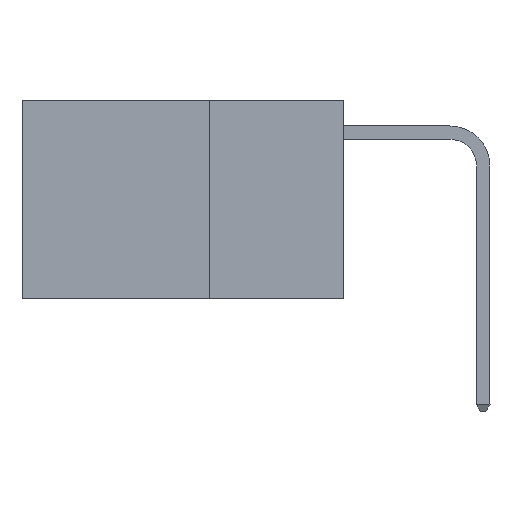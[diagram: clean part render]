
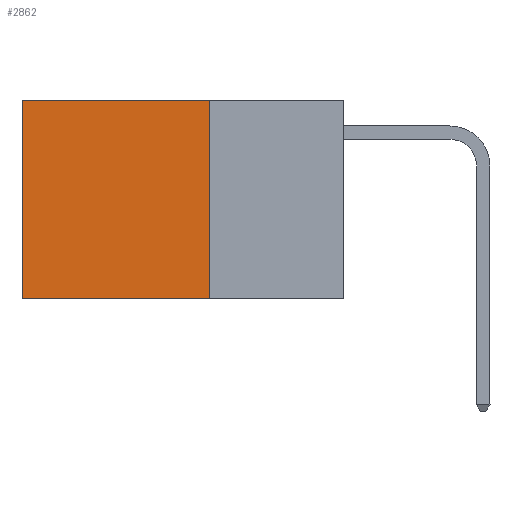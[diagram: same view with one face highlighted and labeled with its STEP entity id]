
A CAD part, left-side view. The second image highlights one B-rep face of the part: STEP entity #2862.
In plain terms, the highlighted planar face has unit normal (-1, 0, 0).
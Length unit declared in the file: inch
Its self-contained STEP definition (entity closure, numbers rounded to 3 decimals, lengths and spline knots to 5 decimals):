
#865 = CARTESIAN_POINT ( 'NONE',  ( 0.2625, 0.6, 0. ) ) ;
#990 = VECTOR ( 'NONE', #8716, 39.37008 ) ;
#1269 = VERTEX_POINT ( 'NONE', #865 ) ;
#1334 = VERTEX_POINT ( 'NONE', #7716 ) ;
#2862 = ADVANCED_FACE ( 'NONE', ( #6163 ), #12573, .F. ) ;
#3674 = EDGE_LOOP ( 'NONE', ( #12179, #13144, #6702, #9783 ) ) ;
#3765 = EDGE_CURVE ( 'NONE', #15240, #1334, #6272, .T. ) ;
#4003 = EDGE_CURVE ( 'NONE', #10254, #1269, #8808, .T. ) ;
#4923 = CARTESIAN_POINT ( 'NONE',  ( 0.2625, 0.25, -0.37 ) ) ;
#5014 = DIRECTION ( 'NONE',  ( 0., 1., 0. ) ) ;
#5397 = VECTOR ( 'NONE', #5014, 39.37008 ) ;
#5686 = LINE ( 'NONE', #14625, #9878 ) ;
#6163 = FACE_OUTER_BOUND ( 'NONE', #3674, .T. ) ;
#6244 = DIRECTION ( 'NONE',  ( 1., 0., 0. ) ) ;
#6272 = LINE ( 'NONE', #4923, #5397 ) ;
#6702 = ORIENTED_EDGE ( 'NONE', *, *, #14490, .F. ) ;
#7448 = CARTESIAN_POINT ( 'NONE',  ( 0.2625, 0.25, 0. ) ) ;
#7615 = DIRECTION ( 'NONE',  ( 0., 0., -1. ) ) ;
#7716 = CARTESIAN_POINT ( 'NONE',  ( 0.2625, 0.6, -0.37 ) ) ;
#8716 = DIRECTION ( 'NONE',  ( 0., 1., 0. ) ) ;
#8808 = LINE ( 'NONE', #13926, #990 ) ;
#9783 = ORIENTED_EDGE ( 'NONE', *, *, #4003, .T. ) ;
#9863 = DIRECTION ( 'NONE',  ( 0., 0., -1. ) ) ;
#9878 = VECTOR ( 'NONE', #13215, 39.37008 ) ;
#10254 = VERTEX_POINT ( 'NONE', #10658 ) ;
#10658 = CARTESIAN_POINT ( 'NONE',  ( 0.2625, 0.25, 0. ) ) ;
#10782 = VECTOR ( 'NONE', #9863, 39.37008 ) ;
#10873 = AXIS2_PLACEMENT_3D ( 'NONE', #7448, #6244, #7615 ) ;
#11032 = EDGE_CURVE ( 'NONE', #1269, #1334, #5686, .T. ) ;
#12179 = ORIENTED_EDGE ( 'NONE', *, *, #11032, .T. ) ;
#12220 = CARTESIAN_POINT ( 'NONE',  ( 0.2625, 0.25, 0. ) ) ;
#12573 = PLANE ( 'NONE',  #10873 ) ;
#13144 = ORIENTED_EDGE ( 'NONE', *, *, #3765, .F. ) ;
#13215 = DIRECTION ( 'NONE',  ( 0., 0., -1. ) ) ;
#13926 = CARTESIAN_POINT ( 'NONE',  ( 0.2625, 0.25, 0. ) ) ;
#14490 = EDGE_CURVE ( 'NONE', #10254, #15240, #15072, .T. ) ;
#14625 = CARTESIAN_POINT ( 'NONE',  ( 0.2625, 0.6, 0. ) ) ;
#15072 = LINE ( 'NONE', #12220, #10782 ) ;
#15240 = VERTEX_POINT ( 'NONE', #15560 ) ;
#15560 = CARTESIAN_POINT ( 'NONE',  ( 0.2625, 0.25, -0.37 ) ) ;
